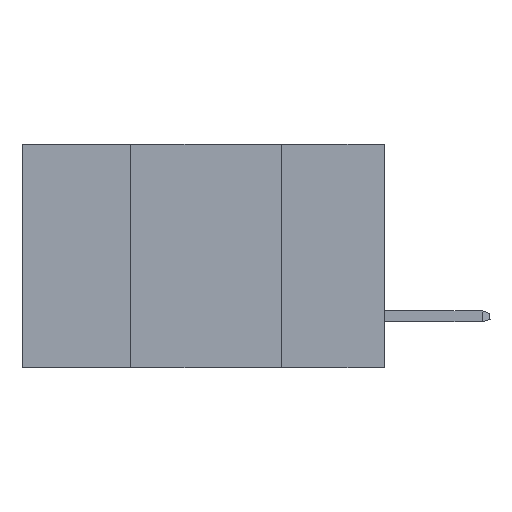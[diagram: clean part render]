
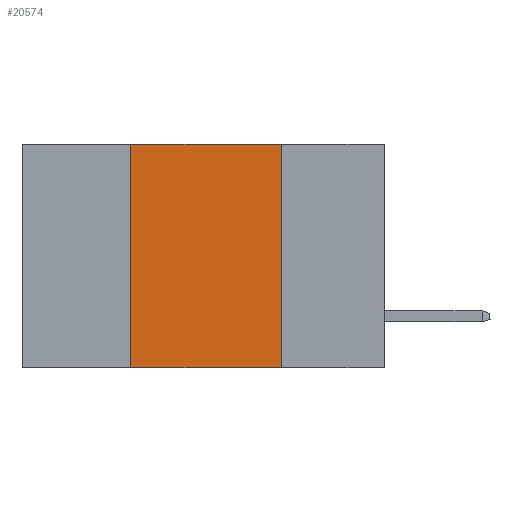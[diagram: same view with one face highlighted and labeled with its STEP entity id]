
A CAD part, left-side view. The second image highlights one B-rep face of the part: STEP entity #20574.
In plain terms, the highlighted planar face has unit normal (-1, 0, 0).
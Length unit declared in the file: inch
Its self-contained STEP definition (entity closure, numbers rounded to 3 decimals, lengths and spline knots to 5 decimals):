
#2078 = DIRECTION ( 'NONE',  ( 0., -1., 0. ) ) ;
#2165 = CARTESIAN_POINT ( 'NONE',  ( 0., 0.6, 0. ) ) ;
#2422 = EDGE_CURVE ( 'NONE', #9140, #13529, #24077, .T. ) ;
#3031 = FACE_OUTER_BOUND ( 'NONE', #21571, .T. ) ;
#4200 = ORIENTED_EDGE ( 'NONE', *, *, #2422, .F. ) ;
#4831 = VECTOR ( 'NONE', #22482, 39.37008 ) ;
#4931 = EDGE_CURVE ( 'NONE', #15617, #9140, #11971, .T. ) ;
#7165 = CARTESIAN_POINT ( 'NONE',  ( 0., 0.42, 0. ) ) ;
#7446 = VECTOR ( 'NONE', #2078, 39.37008 ) ;
#9140 = VERTEX_POINT ( 'NONE', #14706 ) ;
#9725 = DIRECTION ( 'NONE',  ( 0., -1., 0. ) ) ;
#11941 = VERTEX_POINT ( 'NONE', #26486 ) ;
#11971 = LINE ( 'NONE', #2165, #26768 ) ;
#13529 = VERTEX_POINT ( 'NONE', #16308 ) ;
#14706 = CARTESIAN_POINT ( 'NONE',  ( 0., 0.17, 0. ) ) ;
#14930 = ORIENTED_EDGE ( 'NONE', *, *, #22554, .F. ) ;
#15617 = VERTEX_POINT ( 'NONE', #28773 ) ;
#16308 = CARTESIAN_POINT ( 'NONE',  ( 0., 0.17, -0.37 ) ) ;
#17450 = VECTOR ( 'NONE', #25806, 39.37008 ) ;
#17495 = EDGE_CURVE ( 'NONE', #11941, #13529, #29521, .T. ) ;
#18685 = ORIENTED_EDGE ( 'NONE', *, *, #17495, .T. ) ;
#18709 = DIRECTION ( 'NONE',  ( 1., 0., 0. ) ) ;
#18815 = CARTESIAN_POINT ( 'NONE',  ( 0., 0.6, 0. ) ) ;
#20574 = ADVANCED_FACE ( 'NONE', ( #3031 ), #26254, .F. ) ;
#21571 = EDGE_LOOP ( 'NONE', ( #4200, #22586, #14930, #18685 ) ) ;
#22266 = LINE ( 'NONE', #7165, #4831 ) ;
#22482 = DIRECTION ( 'NONE',  ( 0., 0., 1. ) ) ;
#22554 = EDGE_CURVE ( 'NONE', #11941, #15617, #22266, .T. ) ;
#22586 = ORIENTED_EDGE ( 'NONE', *, *, #4931, .F. ) ;
#24077 = LINE ( 'NONE', #28366, #17450 ) ;
#25806 = DIRECTION ( 'NONE',  ( 0., 0., -1. ) ) ;
#26254 = PLANE ( 'NONE',  #29139 ) ;
#26486 = CARTESIAN_POINT ( 'NONE',  ( 0., 0.42, -0.37 ) ) ;
#26768 = VECTOR ( 'NONE', #9725, 39.37008 ) ;
#28366 = CARTESIAN_POINT ( 'NONE',  ( 0., 0.17, 0. ) ) ;
#28706 = DIRECTION ( 'NONE',  ( 0., 0., -1. ) ) ;
#28773 = CARTESIAN_POINT ( 'NONE',  ( 0., 0.42, 0. ) ) ;
#29027 = CARTESIAN_POINT ( 'NONE',  ( 0., 0.6, -0.37 ) ) ;
#29139 = AXIS2_PLACEMENT_3D ( 'NONE', #18815, #18709, #28706 ) ;
#29521 = LINE ( 'NONE', #29027, #7446 ) ;
